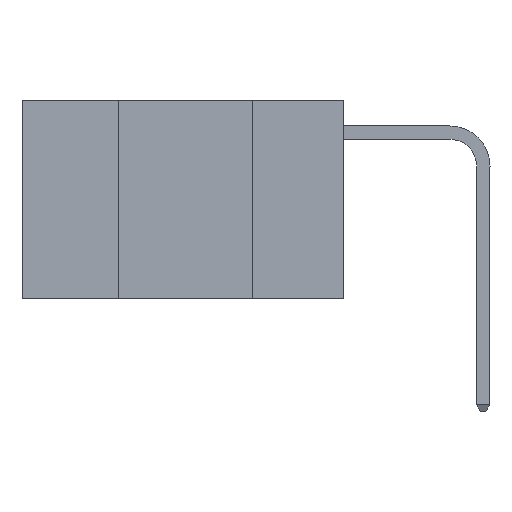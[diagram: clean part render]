
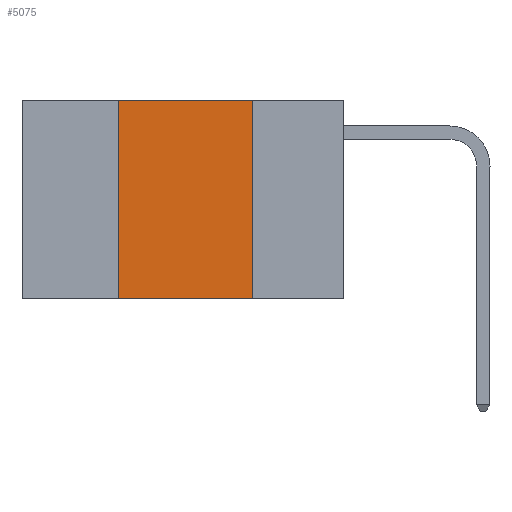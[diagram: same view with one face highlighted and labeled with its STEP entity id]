
A CAD part, left-side view. The second image highlights one B-rep face of the part: STEP entity #5075.
In plain terms, the highlighted planar face has unit normal (-1, 0, 0).
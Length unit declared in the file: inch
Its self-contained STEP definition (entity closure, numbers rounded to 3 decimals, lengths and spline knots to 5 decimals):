
#151 = VECTOR ( 'NONE', #6586, 39.37008 ) ;
#589 = CARTESIAN_POINT ( 'NONE',  ( 0., 0.6, -0.37 ) ) ;
#3011 = CARTESIAN_POINT ( 'NONE',  ( 0., 0.17, 0. ) ) ;
#3414 = CARTESIAN_POINT ( 'NONE',  ( 0., 0.6, 0. ) ) ;
#3446 = VERTEX_POINT ( 'NONE', #6719 ) ;
#3660 = VERTEX_POINT ( 'NONE', #3933 ) ;
#3933 = CARTESIAN_POINT ( 'NONE',  ( 0., 0.42, -0.37 ) ) ;
#4013 = DIRECTION ( 'NONE',  ( 0., -1., 0. ) ) ;
#4213 = FACE_OUTER_BOUND ( 'NONE', #9622, .T. ) ;
#4446 = DIRECTION ( 'NONE',  ( 1., 0., 0. ) ) ;
#4861 = CARTESIAN_POINT ( 'NONE',  ( 0., 0.17, -0.37 ) ) ;
#5075 = ADVANCED_FACE ( 'NONE', ( #4213 ), #9348, .F. ) ;
#5154 = ORIENTED_EDGE ( 'NONE', *, *, #7122, .F. ) ;
#5274 = VERTEX_POINT ( 'NONE', #11536 ) ;
#5320 = ORIENTED_EDGE ( 'NONE', *, *, #7768, .F. ) ;
#5647 = CARTESIAN_POINT ( 'NONE',  ( 0., 0.42, 0. ) ) ;
#5863 = ORIENTED_EDGE ( 'NONE', *, *, #6907, .F. ) ;
#5878 = ORIENTED_EDGE ( 'NONE', *, *, #6884, .T. ) ;
#6572 = VECTOR ( 'NONE', #8652, 39.37008 ) ;
#6586 = DIRECTION ( 'NONE',  ( 0., -1., 0. ) ) ;
#6719 = CARTESIAN_POINT ( 'NONE',  ( 0., 0.42, 0. ) ) ;
#6720 = VECTOR ( 'NONE', #4013, 39.37008 ) ;
#6884 = EDGE_CURVE ( 'NONE', #3660, #9315, #9849, .T. ) ;
#6887 = LINE ( 'NONE', #5647, #6572 ) ;
#6907 = EDGE_CURVE ( 'NONE', #3660, #3446, #6887, .T. ) ;
#7122 = EDGE_CURVE ( 'NONE', #5274, #9315, #12141, .T. ) ;
#7768 = EDGE_CURVE ( 'NONE', #3446, #5274, #9400, .T. ) ;
#7934 = CARTESIAN_POINT ( 'NONE',  ( 0., 0.6, 0. ) ) ;
#8652 = DIRECTION ( 'NONE',  ( 0., 0., 1. ) ) ;
#9095 = VECTOR ( 'NONE', #12667, 39.37008 ) ;
#9315 = VERTEX_POINT ( 'NONE', #4861 ) ;
#9348 = PLANE ( 'NONE',  #10346 ) ;
#9400 = LINE ( 'NONE', #7934, #6720 ) ;
#9622 = EDGE_LOOP ( 'NONE', ( #5154, #5320, #5863, #5878 ) ) ;
#9849 = LINE ( 'NONE', #589, #151 ) ;
#10346 = AXIS2_PLACEMENT_3D ( 'NONE', #3414, #4446, #11216 ) ;
#11216 = DIRECTION ( 'NONE',  ( 0., 0., -1. ) ) ;
#11536 = CARTESIAN_POINT ( 'NONE',  ( 0., 0.17, 0. ) ) ;
#12141 = LINE ( 'NONE', #3011, #9095 ) ;
#12667 = DIRECTION ( 'NONE',  ( 0., 0., -1. ) ) ;
